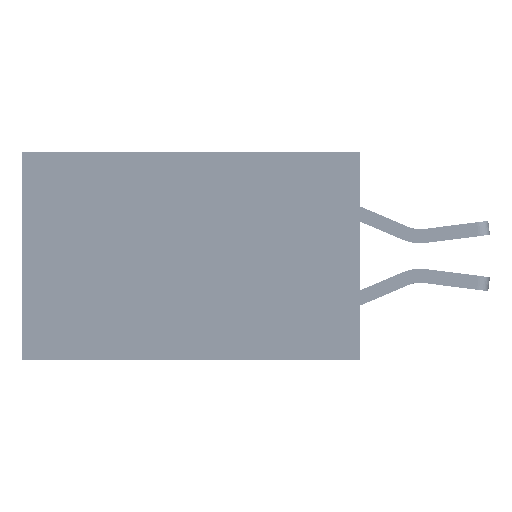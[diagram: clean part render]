
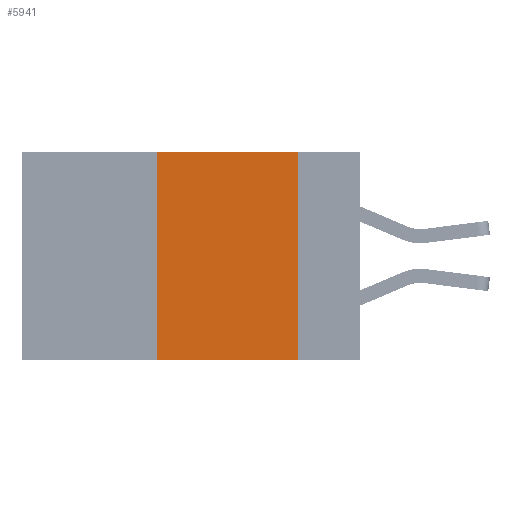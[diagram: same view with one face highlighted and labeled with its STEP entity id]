
A CAD part, left-side view. The second image highlights one B-rep face of the part: STEP entity #5941.
In plain terms, the highlighted planar face has unit normal (-1, 0, 0).
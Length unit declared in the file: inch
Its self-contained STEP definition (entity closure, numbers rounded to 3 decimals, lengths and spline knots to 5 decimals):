
#1264 = PLANE ( 'NONE',  #15518 ) ;
#1431 = DIRECTION ( 'NONE',  ( 0., 0., -1. ) ) ;
#2130 = VECTOR ( 'NONE', #25226, 39.37008 ) ;
#3444 = CARTESIAN_POINT ( 'NONE',  ( 0., 0.11, -0.37 ) ) ;
#4022 = LINE ( 'NONE', #40962, #40451 ) ;
#4404 = DIRECTION ( 'NONE',  ( 0., -1., 0. ) ) ;
#5941 = ADVANCED_FACE ( 'NONE', ( #21327 ), #1264, .F. ) ;
#5943 = CARTESIAN_POINT ( 'NONE',  ( 0., 0.36, 0. ) ) ;
#9961 = ORIENTED_EDGE ( 'NONE', *, *, #11002, .F. ) ;
#10464 = ORIENTED_EDGE ( 'NONE', *, *, #11958, .F. ) ;
#10636 = LINE ( 'NONE', #31432, #2130 ) ;
#11002 = EDGE_CURVE ( 'NONE', #40671, #12169, #4022, .T. ) ;
#11958 = EDGE_CURVE ( 'NONE', #12169, #31947, #32228, .T. ) ;
#12169 = VERTEX_POINT ( 'NONE', #23579 ) ;
#12441 = DIRECTION ( 'NONE',  ( 0., 0., 1. ) ) ;
#13827 = CARTESIAN_POINT ( 'NONE',  ( 0., 0.36, 0. ) ) ;
#15518 = AXIS2_PLACEMENT_3D ( 'NONE', #20757, #30195, #1431 ) ;
#17297 = EDGE_CURVE ( 'NONE', #25893, #31947, #10636, .T. ) ;
#17570 = ORIENTED_EDGE ( 'NONE', *, *, #32569, .F. ) ;
#20757 = CARTESIAN_POINT ( 'NONE',  ( 0., 0.6, 0. ) ) ;
#21327 = FACE_OUTER_BOUND ( 'NONE', #41383, .T. ) ;
#23579 = CARTESIAN_POINT ( 'NONE',  ( 0., 0.11, 0. ) ) ;
#23618 = VECTOR ( 'NONE', #26765, 39.37008 ) ;
#25226 = DIRECTION ( 'NONE',  ( 0., -1., 0. ) ) ;
#25893 = VERTEX_POINT ( 'NONE', #26953 ) ;
#26765 = DIRECTION ( 'NONE',  ( 0., 0., -1. ) ) ;
#26953 = CARTESIAN_POINT ( 'NONE',  ( 0., 0.36, -0.37 ) ) ;
#27299 = ORIENTED_EDGE ( 'NONE', *, *, #17297, .T. ) ;
#28892 = LINE ( 'NONE', #5943, #38486 ) ;
#30195 = DIRECTION ( 'NONE',  ( 1., 0., 0. ) ) ;
#31413 = CARTESIAN_POINT ( 'NONE',  ( 0., 0.11, 0. ) ) ;
#31432 = CARTESIAN_POINT ( 'NONE',  ( 0., 0.6, -0.37 ) ) ;
#31947 = VERTEX_POINT ( 'NONE', #3444 ) ;
#32228 = LINE ( 'NONE', #31413, #23618 ) ;
#32569 = EDGE_CURVE ( 'NONE', #25893, #40671, #28892, .T. ) ;
#38486 = VECTOR ( 'NONE', #12441, 39.37008 ) ;
#40451 = VECTOR ( 'NONE', #4404, 39.37008 ) ;
#40671 = VERTEX_POINT ( 'NONE', #13827 ) ;
#40962 = CARTESIAN_POINT ( 'NONE',  ( 0., 0.6, 0. ) ) ;
#41383 = EDGE_LOOP ( 'NONE', ( #10464, #9961, #17570, #27299 ) ) ;
